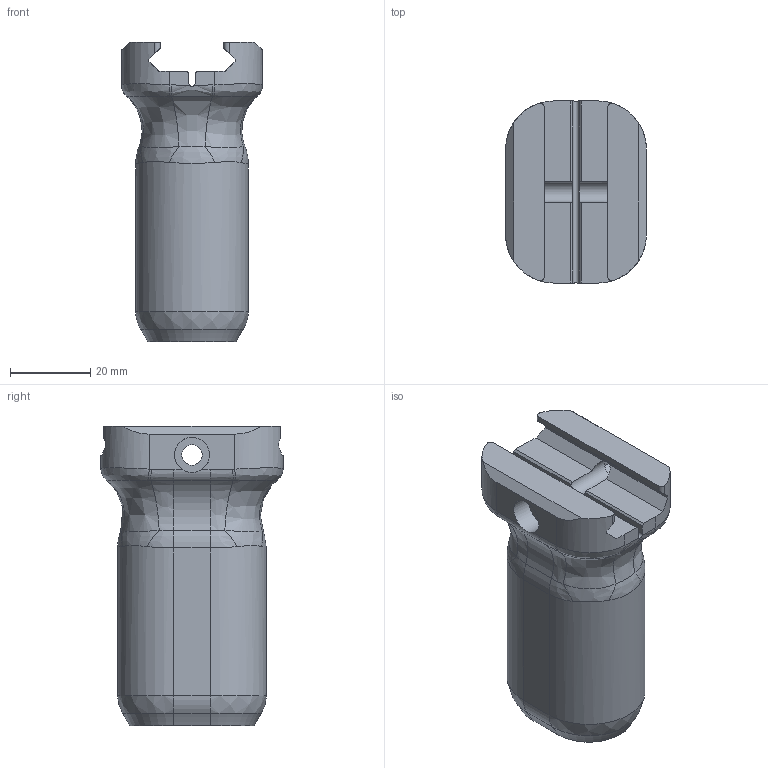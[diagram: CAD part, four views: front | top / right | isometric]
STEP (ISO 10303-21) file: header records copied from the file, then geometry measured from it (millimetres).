
FILE_DESCRIPTION(/* description */ (''),/* implementation_level */ '2;1');
FILE_NAME(/* name */ 'Standard Foregrip.step',/* time_stamp */ '2021-04-06T01:38:38-04:00',/* author */ (''),/* organization */ (''),/* preprocessor_version */ 'ST-DEVELOPER v18.1',/* originating_system */ 'Autodesk Translation Framework v9.10.0.1330',/* authorisation */ '');
FILE_SCHEMA (('AUTOMOTIVE_DESIGN { 1 0 10303 214 3 1 1 }'));
Length unit declared in the file: millimetre
Products named in the file (1): Standard Foregrip
Bounding box: 35 x 45.3 x 74.62 mm (x, y, z)
Volume: 37815.2 mm3; surface area: 16266.7 mm2
Topology: 1 solids, 1 shells, 140 faces, 351 edges, 212 vertices
Faces by surface type: plane 48, bspline 40, cylinder 38, torus 12, cone 2
Full cylindrical faces by diameter (mm): 5.1 x2, 8.75 x1
Entity records: 5287 total; most frequent: CARTESIAN_POINT 2043, ORIENTED_EDGE 702, DIRECTION 635, EDGE_CURVE 351, AXIS2_PLACEMENT_3D 250, VERTEX_POINT 212, EDGE_LOOP 143, FACE_OUTER_BOUND 140
